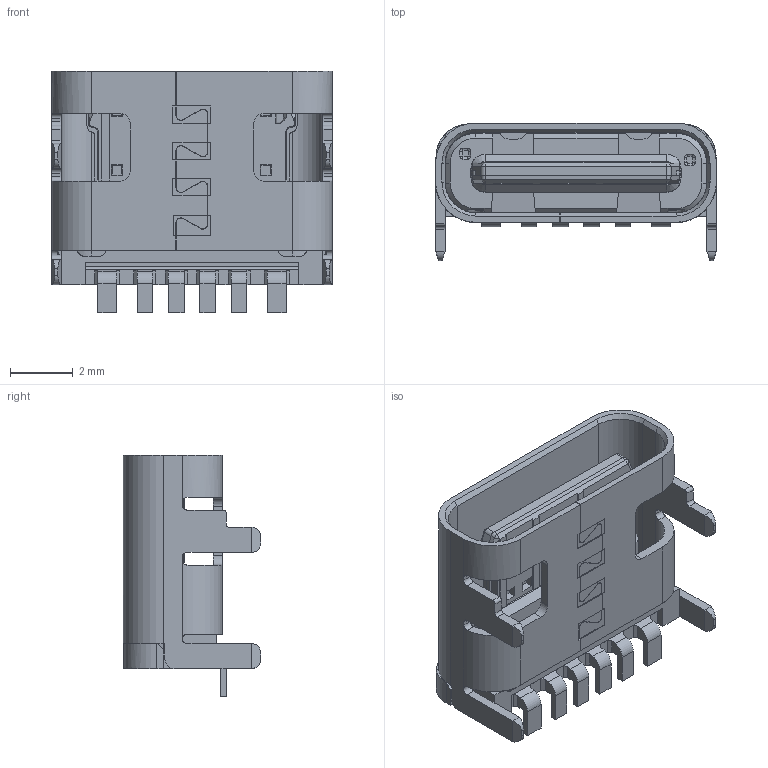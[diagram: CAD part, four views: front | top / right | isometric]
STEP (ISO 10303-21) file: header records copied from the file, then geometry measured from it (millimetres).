
FILE_DESCRIPTION (( 'STEP AP214' ), '1' );
FILE_NAME ('698A106-162-211 - EDAC USB Connector.STEP', '2021-01-15T21:50:50', ( '' ), ( '' ), 'SwSTEP 2.0', 'SolidWorks 2020', '' );
FILE_SCHEMA (( 'AUTOMOTIVE_DESIGN' ));
Length unit declared in the file: millimetre
Products named in the file (3): Insulator 690A06-162-211; Shell 690A106-162-211; 698A106-162-211 - EDAC USB Connector
Assembly tree (2 placements, depth 2):
  698A106-162-211 - EDAC USB Connector
    Insulator 690A06-162-211
    Shell 690A106-162-211
Bounding box: 8.94 x 4.38 x 7.7 mm (x, y, z)
Volume: 91.9 mm3; surface area: 468.1 mm2
Topology: 2 solids, 2 shells, 786 faces, 2139 edges, 1404 vertices
Faces by surface type: plane 595, cylinder 143, cone 28, bspline 20
Entity records: 25776 total; most frequent: CARTESIAN_POINT 5542, ORIENTED_EDGE 4278, DIRECTION 3700, EDGE_CURVE 2139, LINE 1684, VECTOR 1684, VERTEX_POINT 1404, AXIS2_PLACEMENT_3D 1008
